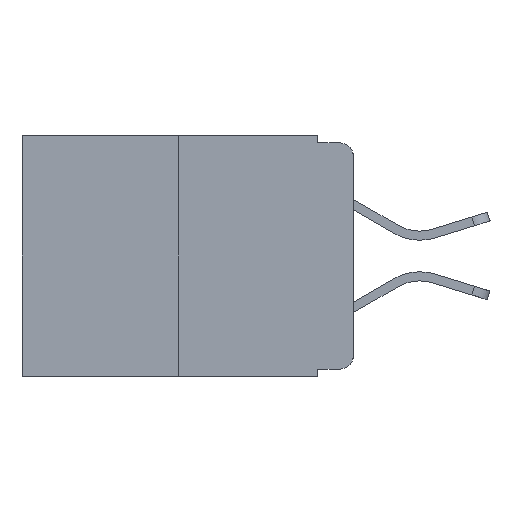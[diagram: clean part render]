
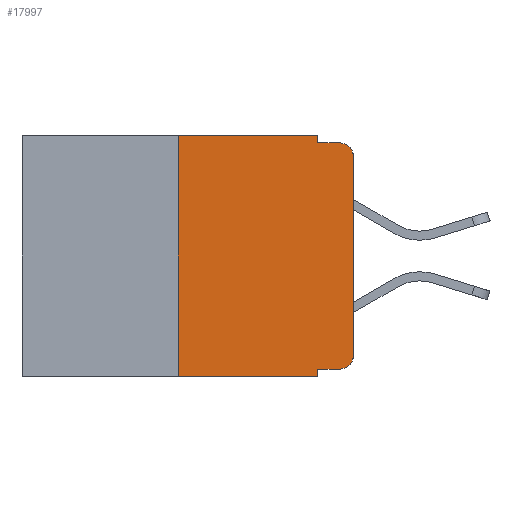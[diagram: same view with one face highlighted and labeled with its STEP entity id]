
A CAD part, left-side view. The second image highlights one B-rep face of the part: STEP entity #17997.
In plain terms, the highlighted planar face has unit normal (-1, 0, 0).
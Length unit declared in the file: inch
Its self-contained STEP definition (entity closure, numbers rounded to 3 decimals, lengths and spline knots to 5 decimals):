
#49 = DIRECTION ( 'NONE',  ( -1., 0., 0. ) ) ;
#179 = CARTESIAN_POINT ( 'NONE',  ( 0., 0.02, -0.313 ) ) ;
#212 = DIRECTION ( 'NONE',  ( -1., 0., 0. ) ) ;
#255 = VERTEX_POINT ( 'NONE', #13909 ) ;
#401 = LINE ( 'NONE', #1598, #1154 ) ;
#792 = VECTOR ( 'NONE', #3775, 39.37008 ) ;
#898 = CARTESIAN_POINT ( 'NONE',  ( 0., 0.051, 0. ) ) ;
#1154 = VECTOR ( 'NONE', #13900, 39.37008 ) ;
#1469 = LINE ( 'NONE', #15473, #9310 ) ;
#1598 = CARTESIAN_POINT ( 'NONE',  ( 0., 0.051, 0. ) ) ;
#1805 = CARTESIAN_POINT ( 'NONE',  ( 0., 0.02, -0.03 ) ) ;
#1857 = EDGE_CURVE ( 'NONE', #11718, #17912, #8401, .T. ) ;
#1935 = ORIENTED_EDGE ( 'NONE', *, *, #7570, .F. ) ;
#2266 = CARTESIAN_POINT ( 'NONE',  ( 0., 0.051, -0.01 ) ) ;
#2434 = EDGE_CURVE ( 'NONE', #5571, #11718, #11826, .T. ) ;
#2579 = CARTESIAN_POINT ( 'NONE',  ( 0., 0.02, -0.01 ) ) ;
#2735 = EDGE_LOOP ( 'NONE', ( #6385, #12396, #14966, #19860, #1935, #11193, #15292, #17839, #11976, #16205 ) ) ;
#3169 = DIRECTION ( 'NONE',  ( 0., -1., 0. ) ) ;
#3567 = AXIS2_PLACEMENT_3D ( 'NONE', #10415, #4067, #15046 ) ;
#3775 = DIRECTION ( 'NONE',  ( 0., -1., 0. ) ) ;
#4067 = DIRECTION ( 'NONE',  ( 1., 0., 0. ) ) ;
#4225 = EDGE_CURVE ( 'NONE', #19554, #10818, #1469, .T. ) ;
#4641 = CARTESIAN_POINT ( 'NONE',  ( 0., 0., 0. ) ) ;
#4806 = CARTESIAN_POINT ( 'NONE',  ( 0., 0.25, 0. ) ) ;
#4821 = CARTESIAN_POINT ( 'NONE',  ( 0., 0.051, -0.343 ) ) ;
#5571 = VERTEX_POINT ( 'NONE', #9112 ) ;
#5619 = EDGE_CURVE ( 'NONE', #17912, #9085, #17559, .T. ) ;
#6238 = VECTOR ( 'NONE', #7101, 39.37008 ) ;
#6385 = ORIENTED_EDGE ( 'NONE', *, *, #5619, .T. ) ;
#6921 = CARTESIAN_POINT ( 'NONE',  ( 0., 0., -0.313 ) ) ;
#7101 = DIRECTION ( 'NONE',  ( 0., -1., 0. ) ) ;
#7275 = DIRECTION ( 'NONE',  ( 0., 0., -1. ) ) ;
#7570 = EDGE_CURVE ( 'NONE', #10818, #17969, #18489, .T. ) ;
#7698 = DIRECTION ( 'NONE',  ( 0., 0., -1. ) ) ;
#8024 = EDGE_CURVE ( 'NONE', #255, #14165, #17738, .T. ) ;
#8293 = VERTEX_POINT ( 'NONE', #4821 ) ;
#8401 = CIRCLE ( 'NONE', #19127, 0.02 ) ;
#9085 = VERTEX_POINT ( 'NONE', #9948 ) ;
#9112 = CARTESIAN_POINT ( 'NONE',  ( 0., 0.051, -0.333 ) ) ;
#9310 = VECTOR ( 'NONE', #19937, 39.37008 ) ;
#9688 = CARTESIAN_POINT ( 'NONE',  ( 0., 0.051, -0.333 ) ) ;
#9948 = CARTESIAN_POINT ( 'NONE',  ( 0., 0., -0.03 ) ) ;
#10415 = CARTESIAN_POINT ( 'NONE',  ( 0., 0.473, 0. ) ) ;
#10663 = VECTOR ( 'NONE', #7275, 39.37008 ) ;
#10684 = CARTESIAN_POINT ( 'NONE',  ( 0., 0.473, 0. ) ) ;
#10818 = VERTEX_POINT ( 'NONE', #4806 ) ;
#10831 = CARTESIAN_POINT ( 'NONE',  ( 0., 0.473, -0.343 ) ) ;
#11193 = ORIENTED_EDGE ( 'NONE', *, *, #4225, .F. ) ;
#11659 = VECTOR ( 'NONE', #12181, 39.37008 ) ;
#11718 = VERTEX_POINT ( 'NONE', #15089 ) ;
#11826 = LINE ( 'NONE', #9688, #792 ) ;
#11976 = ORIENTED_EDGE ( 'NONE', *, *, #2434, .T. ) ;
#12181 = DIRECTION ( 'NONE',  ( 0., -1., 0. ) ) ;
#12396 = ORIENTED_EDGE ( 'NONE', *, *, #16521, .T. ) ;
#13402 = VECTOR ( 'NONE', #20167, 39.37008 ) ;
#13562 = FACE_OUTER_BOUND ( 'NONE', #2735, .T. ) ;
#13701 = CARTESIAN_POINT ( 'NONE',  ( 0., 0.051, 0. ) ) ;
#13900 = DIRECTION ( 'NONE',  ( 0., 0., -1. ) ) ;
#13909 = CARTESIAN_POINT ( 'NONE',  ( 0., 0.051, -0.01 ) ) ;
#14165 = VERTEX_POINT ( 'NONE', #2579 ) ;
#14312 = DIRECTION ( 'NONE',  ( 0., 0., -1. ) ) ;
#14966 = ORIENTED_EDGE ( 'NONE', *, *, #8024, .F. ) ;
#15046 = DIRECTION ( 'NONE',  ( 0., 0., -1. ) ) ;
#15089 = CARTESIAN_POINT ( 'NONE',  ( 0., 0.02, -0.333 ) ) ;
#15292 = ORIENTED_EDGE ( 'NONE', *, *, #17682, .T. ) ;
#15473 = CARTESIAN_POINT ( 'NONE',  ( 0., 0.25, 0. ) ) ;
#15568 = CIRCLE ( 'NONE', #19802, 0.02 ) ;
#16205 = ORIENTED_EDGE ( 'NONE', *, *, #1857, .T. ) ;
#16254 = VECTOR ( 'NONE', #3169, 39.37008 ) ;
#16367 = EDGE_CURVE ( 'NONE', #5571, #8293, #401, .T. ) ;
#16521 = EDGE_CURVE ( 'NONE', #9085, #14165, #15568, .T. ) ;
#17418 = EDGE_CURVE ( 'NONE', #17969, #255, #18716, .T. ) ;
#17559 = LINE ( 'NONE', #4641, #13402 ) ;
#17682 = EDGE_CURVE ( 'NONE', #19554, #8293, #19948, .T. ) ;
#17738 = LINE ( 'NONE', #2266, #6238 ) ;
#17839 = ORIENTED_EDGE ( 'NONE', *, *, #16367, .F. ) ;
#17912 = VERTEX_POINT ( 'NONE', #6921 ) ;
#17969 = VERTEX_POINT ( 'NONE', #898 ) ;
#17997 = ADVANCED_FACE ( 'NONE', ( #13562 ), #18120, .F. ) ;
#18120 = PLANE ( 'NONE',  #3567 ) ;
#18489 = LINE ( 'NONE', #10684, #11659 ) ;
#18716 = LINE ( 'NONE', #13701, #10663 ) ;
#19127 = AXIS2_PLACEMENT_3D ( 'NONE', #179, #49, #7698 ) ;
#19554 = VERTEX_POINT ( 'NONE', #20056 ) ;
#19802 = AXIS2_PLACEMENT_3D ( 'NONE', #1805, #212, #14312 ) ;
#19860 = ORIENTED_EDGE ( 'NONE', *, *, #17418, .F. ) ;
#19937 = DIRECTION ( 'NONE',  ( 0., 0., 1. ) ) ;
#19948 = LINE ( 'NONE', #10831, #16254 ) ;
#20056 = CARTESIAN_POINT ( 'NONE',  ( 0., 0.25, -0.343 ) ) ;
#20167 = DIRECTION ( 'NONE',  ( 0., 0., 1. ) ) ;
